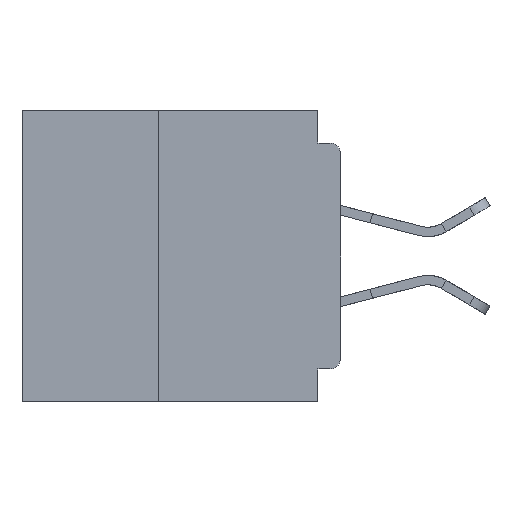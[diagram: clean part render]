
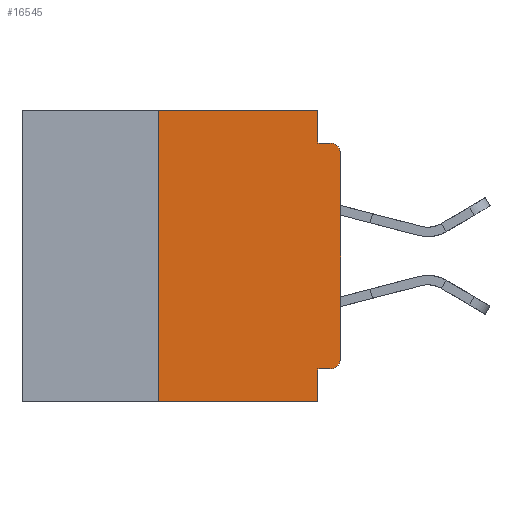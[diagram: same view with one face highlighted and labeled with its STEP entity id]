
A CAD part, left-side view. The second image highlights one B-rep face of the part: STEP entity #16545.
In plain terms, the highlighted planar face has unit normal (-1, 0, 0).
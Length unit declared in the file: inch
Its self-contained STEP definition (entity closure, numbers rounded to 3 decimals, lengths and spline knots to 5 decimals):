
#604 = AXIS2_PLACEMENT_3D ( 'NONE', #5515, #26445, #8505 ) ;
#933 = ORIENTED_EDGE ( 'NONE', *, *, #28561, .F. ) ;
#1289 = CARTESIAN_POINT ( 'NONE',  ( 0., 0.031, -0.4 ) ) ;
#1301 = CARTESIAN_POINT ( 'NONE',  ( 0., 0.437, 0. ) ) ;
#1577 = AXIS2_PLACEMENT_3D ( 'NONE', #28955, #11058, #31840 ) ;
#1646 = DIRECTION ( 'NONE',  ( 0., -1., 0. ) ) ;
#2074 = CARTESIAN_POINT ( 'NONE',  ( 0., 0.015, -0.045 ) ) ;
#2126 = VECTOR ( 'NONE', #37696, 39.37008 ) ;
#2183 = CARTESIAN_POINT ( 'NONE',  ( 0., 0., -0.06 ) ) ;
#3654 = CARTESIAN_POINT ( 'NONE',  ( 0., 0.031, 0. ) ) ;
#4967 = EDGE_CURVE ( 'NONE', #25638, #36698, #8674, .T. ) ;
#5193 = EDGE_CURVE ( 'NONE', #25054, #10090, #26067, .T. ) ;
#5515 = CARTESIAN_POINT ( 'NONE',  ( 0., 0.015, -0.34 ) ) ;
#5577 = ORIENTED_EDGE ( 'NONE', *, *, #5193, .F. ) ;
#6017 = VERTEX_POINT ( 'NONE', #30541 ) ;
#7557 = ORIENTED_EDGE ( 'NONE', *, *, #11843, .T. ) ;
#7826 = CIRCLE ( 'NONE', #1577, 0.015 ) ;
#8505 = DIRECTION ( 'NONE',  ( 0., 0., -1. ) ) ;
#8674 = LINE ( 'NONE', #1301, #15611 ) ;
#9484 = DIRECTION ( 'NONE',  ( 0., 0., -1. ) ) ;
#9768 = DIRECTION ( 'NONE',  ( 0., 0., -1. ) ) ;
#9885 = ORIENTED_EDGE ( 'NONE', *, *, #13249, .F. ) ;
#10006 = VECTOR ( 'NONE', #33557, 39.37008 ) ;
#10090 = VERTEX_POINT ( 'NONE', #2074 ) ;
#10454 = EDGE_CURVE ( 'NONE', #36698, #25054, #16765, .T. ) ;
#10625 = LINE ( 'NONE', #27421, #26610 ) ;
#11058 = DIRECTION ( 'NONE',  ( -1., 0., 0. ) ) ;
#11230 = EDGE_CURVE ( 'NONE', #17143, #20601, #10625, .T. ) ;
#11633 = ORIENTED_EDGE ( 'NONE', *, *, #10454, .F. ) ;
#11843 = EDGE_CURVE ( 'NONE', #6017, #20601, #23825, .T. ) ;
#12050 = ORIENTED_EDGE ( 'NONE', *, *, #34507, .T. ) ;
#12604 = CARTESIAN_POINT ( 'NONE',  ( 0., 0.437, 0. ) ) ;
#13094 = AXIS2_PLACEMENT_3D ( 'NONE', #12604, #36202, #18629 ) ;
#13111 = CARTESIAN_POINT ( 'NONE',  ( 0., 0., -0.34 ) ) ;
#13249 = EDGE_CURVE ( 'NONE', #25641, #17143, #34545, .T. ) ;
#14536 = VECTOR ( 'NONE', #37910, 39.37008 ) ;
#14849 = FACE_OUTER_BOUND ( 'NONE', #15571, .T. ) ;
#15394 = CARTESIAN_POINT ( 'NONE',  ( 0., 0., 0. ) ) ;
#15571 = EDGE_LOOP ( 'NONE', ( #26592, #12050, #5577, #11633, #20113, #933, #7557, #33949, #9885, #20674 ) ) ;
#15572 = PLANE ( 'NONE',  #13094 ) ;
#15611 = VECTOR ( 'NONE', #1646, 39.37008 ) ;
#15821 = VECTOR ( 'NONE', #9768, 39.37008 ) ;
#16545 = ADVANCED_FACE ( 'NONE', ( #14849 ), #15572, .F. ) ;
#16711 = VECTOR ( 'NONE', #27500, 39.37008 ) ;
#16765 = LINE ( 'NONE', #33456, #15821 ) ;
#17143 = VERTEX_POINT ( 'NONE', #36173 ) ;
#17315 = CARTESIAN_POINT ( 'NONE',  ( 0., 0.015, -0.355 ) ) ;
#17654 = LINE ( 'NONE', #15394, #16711 ) ;
#17667 = EDGE_CURVE ( 'NONE', #23649, #25024, #17654, .T. ) ;
#18097 = EDGE_CURVE ( 'NONE', #25641, #23649, #28414, .T. ) ;
#18629 = DIRECTION ( 'NONE',  ( 0., 0., -1. ) ) ;
#20113 = ORIENTED_EDGE ( 'NONE', *, *, #4967, .F. ) ;
#20261 = CARTESIAN_POINT ( 'NONE',  ( 0., 0.031, -0.045 ) ) ;
#20601 = VERTEX_POINT ( 'NONE', #1289 ) ;
#20674 = ORIENTED_EDGE ( 'NONE', *, *, #18097, .T. ) ;
#22659 = LINE ( 'NONE', #26370, #14536 ) ;
#23318 = CARTESIAN_POINT ( 'NONE',  ( 0., 0., -0.045 ) ) ;
#23344 = CARTESIAN_POINT ( 'NONE',  ( 0., 0.25, 0. ) ) ;
#23649 = VERTEX_POINT ( 'NONE', #13111 ) ;
#23825 = LINE ( 'NONE', #24699, #36457 ) ;
#24699 = CARTESIAN_POINT ( 'NONE',  ( 0., 0.437, -0.4 ) ) ;
#25024 = VERTEX_POINT ( 'NONE', #2183 ) ;
#25054 = VERTEX_POINT ( 'NONE', #20261 ) ;
#25638 = VERTEX_POINT ( 'NONE', #23344 ) ;
#25641 = VERTEX_POINT ( 'NONE', #17315 ) ;
#26067 = LINE ( 'NONE', #23318, #2126 ) ;
#26370 = CARTESIAN_POINT ( 'NONE',  ( 0., 0.25, -0.4 ) ) ;
#26445 = DIRECTION ( 'NONE',  ( -1., 0., 0. ) ) ;
#26592 = ORIENTED_EDGE ( 'NONE', *, *, #17667, .T. ) ;
#26610 = VECTOR ( 'NONE', #9484, 39.37008 ) ;
#27421 = CARTESIAN_POINT ( 'NONE',  ( 0., 0.031, -0.4 ) ) ;
#27500 = DIRECTION ( 'NONE',  ( 0., 0., 1. ) ) ;
#27789 = CARTESIAN_POINT ( 'NONE',  ( 0., 0., -0.355 ) ) ;
#28414 = CIRCLE ( 'NONE', #604, 0.015 ) ;
#28561 = EDGE_CURVE ( 'NONE', #6017, #25638, #22659, .T. ) ;
#28955 = CARTESIAN_POINT ( 'NONE',  ( 0., 0.015, -0.06 ) ) ;
#30541 = CARTESIAN_POINT ( 'NONE',  ( 0., 0.25, -0.4 ) ) ;
#31840 = DIRECTION ( 'NONE',  ( 0., 0., -1. ) ) ;
#33456 = CARTESIAN_POINT ( 'NONE',  ( 0., 0.031, 0. ) ) ;
#33557 = DIRECTION ( 'NONE',  ( 0., 1., 0. ) ) ;
#33949 = ORIENTED_EDGE ( 'NONE', *, *, #11230, .F. ) ;
#34507 = EDGE_CURVE ( 'NONE', #25024, #10090, #7826, .T. ) ;
#34545 = LINE ( 'NONE', #27789, #10006 ) ;
#36173 = CARTESIAN_POINT ( 'NONE',  ( 0., 0.031, -0.355 ) ) ;
#36202 = DIRECTION ( 'NONE',  ( 1., 0., 0. ) ) ;
#36284 = DIRECTION ( 'NONE',  ( 0., -1., 0. ) ) ;
#36457 = VECTOR ( 'NONE', #36284, 39.37008 ) ;
#36698 = VERTEX_POINT ( 'NONE', #3654 ) ;
#37696 = DIRECTION ( 'NONE',  ( 0., -1., 0. ) ) ;
#37910 = DIRECTION ( 'NONE',  ( 0., 0., 1. ) ) ;
